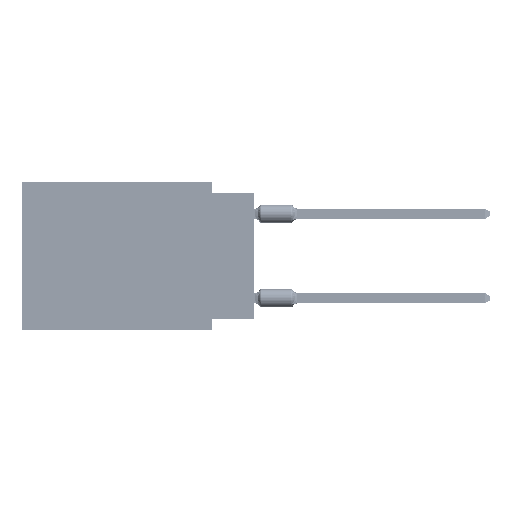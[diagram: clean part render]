
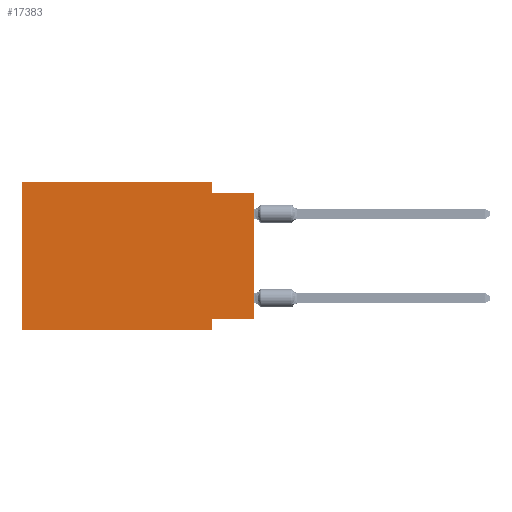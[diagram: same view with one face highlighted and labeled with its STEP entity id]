
A CAD part, left-side view. The second image highlights one B-rep face of the part: STEP entity #17383.
In plain terms, the highlighted planar face has unit normal (-1, 0, 0).
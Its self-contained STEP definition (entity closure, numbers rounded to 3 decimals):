
#774 = ORIENTED_EDGE ( 'NONE', *, *, #10888, .F. ) ;
#4035 = EDGE_CURVE ( 'NONE', #6206, #5110, #9465, .T. ) ;
#5110 = VERTEX_POINT ( 'NONE', #42362 ) ;
#5825 = DIRECTION ( 'NONE',  ( 0., -1., 0. ) ) ;
#6101 = VERTEX_POINT ( 'NONE', #10387 ) ;
#6206 = VERTEX_POINT ( 'NONE', #11091 ) ;
#7119 = PLANE ( 'NONE',  #49870 ) ;
#9465 = LINE ( 'NONE', #21135, #20231 ) ;
#9834 = CARTESIAN_POINT ( 'NONE',  ( 0., 0., -0.635 ) ) ;
#10387 = CARTESIAN_POINT ( 'NONE',  ( 0., 13.97, 0. ) ) ;
#10574 = VECTOR ( 'NONE', #54820, 1000. ) ;
#10888 = EDGE_CURVE ( 'NONE', #31449, #12002, #57868, .T. ) ;
#11091 = CARTESIAN_POINT ( 'NONE',  ( 0., 2.54, -8.255 ) ) ;
#11286 = LINE ( 'NONE', #33584, #72134 ) ;
#12002 = VERTEX_POINT ( 'NONE', #42519 ) ;
#13543 = ORIENTED_EDGE ( 'NONE', *, *, #56189, .T. ) ;
#14301 = EDGE_CURVE ( 'NONE', #6101, #31449, #47671, .T. ) ;
#14800 = LINE ( 'NONE', #59726, #71143 ) ;
#14918 = CARTESIAN_POINT ( 'NONE',  ( 0., 0., -8.255 ) ) ;
#15458 = EDGE_LOOP ( 'NONE', ( #37189, #41697, #774, #43142, #25667, #13543, #48639, #38914 ) ) ;
#15571 = EDGE_CURVE ( 'NONE', #26277, #6206, #43034, .T. ) ;
#15760 = VECTOR ( 'NONE', #35273, 1000. ) ;
#17383 = ADVANCED_FACE ( 'NONE', ( #40351 ), #7119, .F. ) ;
#20231 = VECTOR ( 'NONE', #37935, 1000. ) ;
#20815 = VERTEX_POINT ( 'NONE', #61409 ) ;
#21135 = CARTESIAN_POINT ( 'NONE',  ( 0., 2.54, -8.89 ) ) ;
#21504 = EDGE_CURVE ( 'NONE', #20815, #6101, #14800, .T. ) ;
#24642 = DIRECTION ( 'NONE',  ( 0., 0., -1. ) ) ;
#25667 = ORIENTED_EDGE ( 'NONE', *, *, #21504, .F. ) ;
#26277 = VERTEX_POINT ( 'NONE', #57714 ) ;
#27989 = LINE ( 'NONE', #54667, #64445 ) ;
#31449 = VERTEX_POINT ( 'NONE', #31991 ) ;
#31991 = CARTESIAN_POINT ( 'NONE',  ( 0., 2.54, 0. ) ) ;
#33584 = CARTESIAN_POINT ( 'NONE',  ( 0., 13.97, -8.89 ) ) ;
#35273 = DIRECTION ( 'NONE',  ( 0., -1., 0. ) ) ;
#36887 = VECTOR ( 'NONE', #71164, 1000. ) ;
#37084 = DIRECTION ( 'NONE',  ( 0., 0., 1. ) ) ;
#37189 = ORIENTED_EDGE ( 'NONE', *, *, #62276, .T. ) ;
#37935 = DIRECTION ( 'NONE',  ( 0., 0., -1. ) ) ;
#38914 = ORIENTED_EDGE ( 'NONE', *, *, #15571, .F. ) ;
#40351 = FACE_OUTER_BOUND ( 'NONE', #15458, .T. ) ;
#41082 = CARTESIAN_POINT ( 'NONE',  ( 0., 13.97, 0. ) ) ;
#41601 = VECTOR ( 'NONE', #62631, 1000. ) ;
#41697 = ORIENTED_EDGE ( 'NONE', *, *, #58874, .F. ) ;
#42362 = CARTESIAN_POINT ( 'NONE',  ( 0., 2.54, -8.89 ) ) ;
#42519 = CARTESIAN_POINT ( 'NONE',  ( 0., 2.54, -0.635 ) ) ;
#43034 = LINE ( 'NONE', #14918, #36887 ) ;
#43142 = ORIENTED_EDGE ( 'NONE', *, *, #14301, .F. ) ;
#46592 = CARTESIAN_POINT ( 'NONE',  ( 0., 13.97, 0. ) ) ;
#47260 = CARTESIAN_POINT ( 'NONE',  ( 0., 2.54, 0. ) ) ;
#47671 = LINE ( 'NONE', #46592, #15760 ) ;
#48639 = ORIENTED_EDGE ( 'NONE', *, *, #4035, .F. ) ;
#49338 = CARTESIAN_POINT ( 'NONE',  ( 0., 0., -0.635 ) ) ;
#49870 = AXIS2_PLACEMENT_3D ( 'NONE', #41082, #62642, #24642 ) ;
#50415 = LINE ( 'NONE', #49338, #10574 ) ;
#54667 = CARTESIAN_POINT ( 'NONE',  ( 0., 0., 0. ) ) ;
#54820 = DIRECTION ( 'NONE',  ( 0., -1., 0. ) ) ;
#56189 = EDGE_CURVE ( 'NONE', #20815, #5110, #11286, .T. ) ;
#57714 = CARTESIAN_POINT ( 'NONE',  ( 0., 0., -8.255 ) ) ;
#57868 = LINE ( 'NONE', #47260, #41601 ) ;
#58874 = EDGE_CURVE ( 'NONE', #12002, #61718, #50415, .T. ) ;
#59726 = CARTESIAN_POINT ( 'NONE',  ( 0., 13.97, 0. ) ) ;
#61409 = CARTESIAN_POINT ( 'NONE',  ( 0., 13.97, -8.89 ) ) ;
#61718 = VERTEX_POINT ( 'NONE', #9834 ) ;
#62276 = EDGE_CURVE ( 'NONE', #26277, #61718, #27989, .T. ) ;
#62631 = DIRECTION ( 'NONE',  ( 0., 0., -1. ) ) ;
#62642 = DIRECTION ( 'NONE',  ( 1., 0., 0. ) ) ;
#64445 = VECTOR ( 'NONE', #65992, 1000. ) ;
#65992 = DIRECTION ( 'NONE',  ( 0., 0., 1. ) ) ;
#71143 = VECTOR ( 'NONE', #37084, 1000. ) ;
#71164 = DIRECTION ( 'NONE',  ( 0., 1., 0. ) ) ;
#72134 = VECTOR ( 'NONE', #5825, 1000. ) ;
